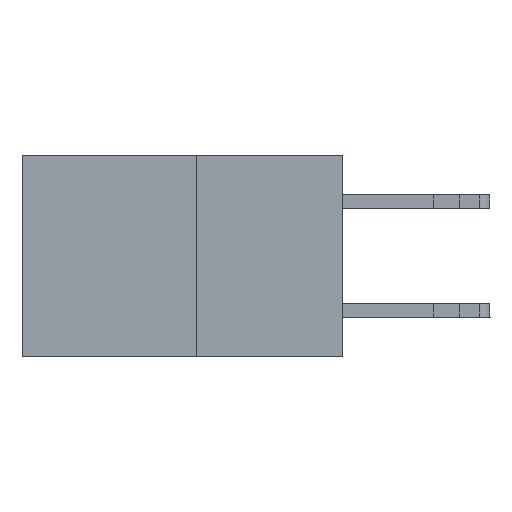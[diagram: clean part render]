
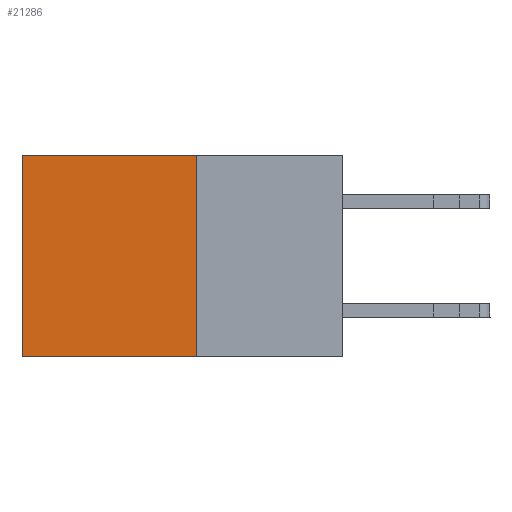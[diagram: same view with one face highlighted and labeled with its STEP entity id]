
A CAD part, left-side view. The second image highlights one B-rep face of the part: STEP entity #21286.
In plain terms, the highlighted planar face has unit normal (-1, 0, 0).
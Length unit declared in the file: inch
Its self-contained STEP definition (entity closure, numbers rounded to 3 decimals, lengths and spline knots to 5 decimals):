
#14 = LINE ( 'NONE', #11906, #25169 ) ;
#493 = LINE ( 'NONE', #15537, #5469 ) ;
#2668 = DIRECTION ( 'NONE',  ( 0., 0., -1. ) ) ;
#3679 = VERTEX_POINT ( 'NONE', #12338 ) ;
#4039 = DIRECTION ( 'NONE',  ( 0., 0., -1. ) ) ;
#4202 = AXIS2_PLACEMENT_3D ( 'NONE', #16266, #18700, #4039 ) ;
#5465 = DIRECTION ( 'NONE',  ( 0., 0., -1. ) ) ;
#5469 = VECTOR ( 'NONE', #30019, 39.37008 ) ;
#5712 = ORIENTED_EDGE ( 'NONE', *, *, #20923, .T. ) ;
#6349 = VERTEX_POINT ( 'NONE', #13692 ) ;
#7077 = DIRECTION ( 'NONE',  ( 0., 1., 0. ) ) ;
#7992 = EDGE_LOOP ( 'NONE', ( #5712, #20384, #27518, #20712 ) ) ;
#10889 = LINE ( 'NONE', #29666, #22253 ) ;
#10893 = CARTESIAN_POINT ( 'NONE',  ( 0.277, 0.59, 0. ) ) ;
#11507 = EDGE_CURVE ( 'NONE', #6349, #18468, #14, .T. ) ;
#11906 = CARTESIAN_POINT ( 'NONE',  ( 0.277, 0.27, 0. ) ) ;
#12338 = CARTESIAN_POINT ( 'NONE',  ( 0.277, 0.59, -0.37 ) ) ;
#13692 = CARTESIAN_POINT ( 'NONE',  ( 0.277, 0.27, 0. ) ) ;
#13812 = PLANE ( 'NONE',  #4202 ) ;
#14908 = CARTESIAN_POINT ( 'NONE',  ( 0.277, 0.59, -0.37 ) ) ;
#15537 = CARTESIAN_POINT ( 'NONE',  ( 0.277, 0.27, -0.37 ) ) ;
#16210 = EDGE_CURVE ( 'NONE', #23758, #3679, #493, .T. ) ;
#16266 = CARTESIAN_POINT ( 'NONE',  ( 0.277, 0.27, -0.37 ) ) ;
#17633 = VECTOR ( 'NONE', #2668, 39.37008 ) ;
#18468 = VERTEX_POINT ( 'NONE', #10893 ) ;
#18700 = DIRECTION ( 'NONE',  ( 1., 0., 0. ) ) ;
#20384 = ORIENTED_EDGE ( 'NONE', *, *, #16210, .F. ) ;
#20712 = ORIENTED_EDGE ( 'NONE', *, *, #11507, .T. ) ;
#20923 = EDGE_CURVE ( 'NONE', #18468, #3679, #24062, .T. ) ;
#21286 = ADVANCED_FACE ( 'NONE', ( #25564 ), #13812, .F. ) ;
#22253 = VECTOR ( 'NONE', #5465, 39.37008 ) ;
#22398 = CARTESIAN_POINT ( 'NONE',  ( 0.277, 0.27, -0.37 ) ) ;
#23758 = VERTEX_POINT ( 'NONE', #22398 ) ;
#24062 = LINE ( 'NONE', #14908, #17633 ) ;
#25169 = VECTOR ( 'NONE', #7077, 39.37008 ) ;
#25564 = FACE_OUTER_BOUND ( 'NONE', #7992, .T. ) ;
#27071 = EDGE_CURVE ( 'NONE', #6349, #23758, #10889, .T. ) ;
#27518 = ORIENTED_EDGE ( 'NONE', *, *, #27071, .F. ) ;
#29666 = CARTESIAN_POINT ( 'NONE',  ( 0.277, 0.27, -0.37 ) ) ;
#30019 = DIRECTION ( 'NONE',  ( 0., 1., 0. ) ) ;
